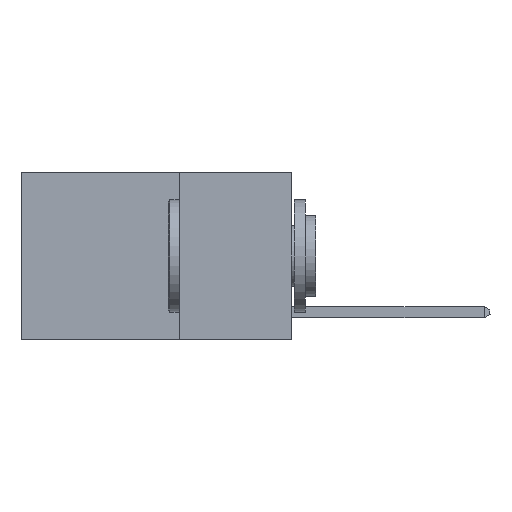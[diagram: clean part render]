
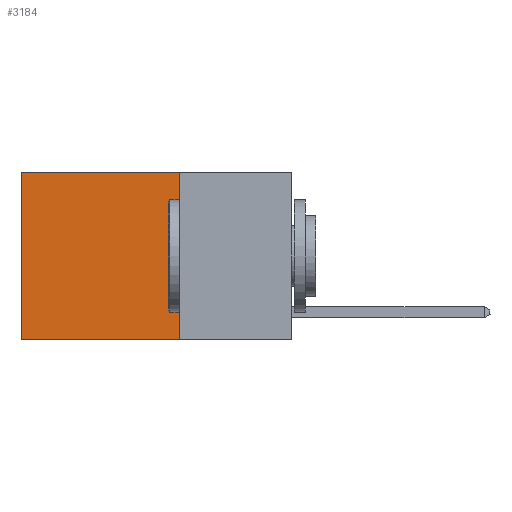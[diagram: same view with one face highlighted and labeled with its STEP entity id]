
A CAD part, left-side view. The second image highlights one B-rep face of the part: STEP entity #3184.
In plain terms, the highlighted planar face has unit normal (-1, 0, 0).
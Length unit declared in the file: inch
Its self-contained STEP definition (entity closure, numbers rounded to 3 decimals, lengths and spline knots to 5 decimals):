
#520 = DIRECTION ( 'NONE',  ( 0., 0., -1. ) ) ;
#682 = LINE ( 'NONE', #12352, #4335 ) ;
#740 = DIRECTION ( 'NONE',  ( 0., 1., 0. ) ) ;
#977 = CARTESIAN_POINT ( 'NONE',  ( 0.2625, 0.25, -0.37 ) ) ;
#986 = AXIS2_PLACEMENT_3D ( 'NONE', #10989, #1638, #9694 ) ;
#1638 = DIRECTION ( 'NONE',  ( 1., 0., 0. ) ) ;
#1802 = FACE_OUTER_BOUND ( 'NONE', #13642, .T. ) ;
#2454 = VECTOR ( 'NONE', #4850, 39.37008 ) ;
#3184 = ADVANCED_FACE ( 'NONE', ( #1802 ), #16284, .F. ) ;
#3314 = ORIENTED_EDGE ( 'NONE', *, *, #11871, .T. ) ;
#3340 = VERTEX_POINT ( 'NONE', #4977 ) ;
#4132 = ORIENTED_EDGE ( 'NONE', *, *, #8901, .T. ) ;
#4335 = VECTOR ( 'NONE', #520, 39.37008 ) ;
#4487 = VERTEX_POINT ( 'NONE', #14996 ) ;
#4582 = CARTESIAN_POINT ( 'NONE',  ( 0.2625, 0.6, -0.37 ) ) ;
#4850 = DIRECTION ( 'NONE',  ( 0., 1., 0. ) ) ;
#4977 = CARTESIAN_POINT ( 'NONE',  ( 0.2625, 0.25, -0.37 ) ) ;
#5562 = ORIENTED_EDGE ( 'NONE', *, *, #14547, .F. ) ;
#7335 = DIRECTION ( 'NONE',  ( 0., 0., -1. ) ) ;
#7507 = VECTOR ( 'NONE', #740, 39.37008 ) ;
#8474 = EDGE_CURVE ( 'NONE', #14647, #3340, #12441, .T. ) ;
#8901 = EDGE_CURVE ( 'NONE', #14647, #4487, #10203, .T. ) ;
#9694 = DIRECTION ( 'NONE',  ( 0., 0., -1. ) ) ;
#9942 = CARTESIAN_POINT ( 'NONE',  ( 0.2625, 0.25, 0. ) ) ;
#10203 = LINE ( 'NONE', #9942, #7507 ) ;
#10989 = CARTESIAN_POINT ( 'NONE',  ( 0.2625, 0.25, 0. ) ) ;
#11871 = EDGE_CURVE ( 'NONE', #4487, #16001, #682, .T. ) ;
#12075 = ORIENTED_EDGE ( 'NONE', *, *, #8474, .F. ) ;
#12352 = CARTESIAN_POINT ( 'NONE',  ( 0.2625, 0.6, 0. ) ) ;
#12441 = LINE ( 'NONE', #13639, #15081 ) ;
#13639 = CARTESIAN_POINT ( 'NONE',  ( 0.2625, 0.25, 0. ) ) ;
#13642 = EDGE_LOOP ( 'NONE', ( #3314, #5562, #12075, #4132 ) ) ;
#14428 = CARTESIAN_POINT ( 'NONE',  ( 0.2625, 0.25, 0. ) ) ;
#14547 = EDGE_CURVE ( 'NONE', #3340, #16001, #15403, .T. ) ;
#14647 = VERTEX_POINT ( 'NONE', #14428 ) ;
#14996 = CARTESIAN_POINT ( 'NONE',  ( 0.2625, 0.6, 0. ) ) ;
#15081 = VECTOR ( 'NONE', #7335, 39.37008 ) ;
#15403 = LINE ( 'NONE', #977, #2454 ) ;
#16001 = VERTEX_POINT ( 'NONE', #4582 ) ;
#16284 = PLANE ( 'NONE',  #986 ) ;
